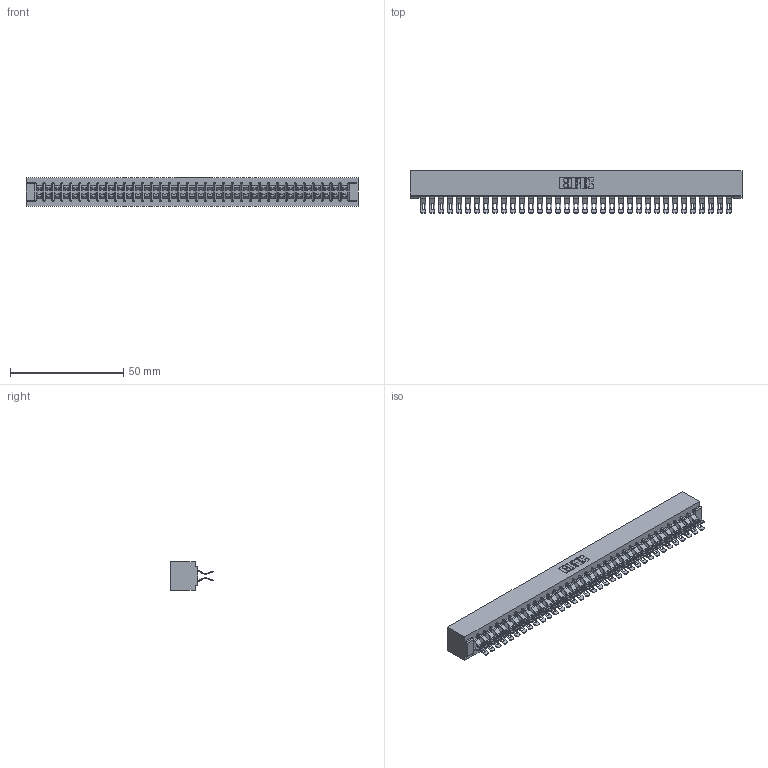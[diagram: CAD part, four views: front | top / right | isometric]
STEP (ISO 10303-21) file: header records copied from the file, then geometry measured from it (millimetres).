
FILE_DESCRIPTION (( 'STEP AP203' ), '1' );
FILE_NAME ('357-070-455-201.STEP', '2020-10-04T21:39:16', ( '' ), ( '' ), 'SwSTEP 2.0', 'SolidWorks 2020', '' );
FILE_SCHEMA (( 'CONFIG_CONTROL_DESIGN' ));
Length unit declared in the file: inch
Products named in the file (3): 307-290-001_555; 307 Part_No Mounting Lugs; 357-070-455-201
Assembly tree (71 placements, depth 2):
  357-070-455-201
    307 Part_No Mounting Lugs
    307-290-001_555  x70
Bounding box: 146.56 x 18.75 x 12.7 mm (x, y, z)
Volume: 16291.2 mm3; surface area: 21264.4 mm2
Topology: 71 solids, 71 shells, 4416 faces, 12969 edges, 8454 vertices
Faces by surface type: plane 2446, cylinder 1898, sphere 72
Entity records: 32247 total; most frequent: CARTESIAN_POINT 5279, ORIENTED_EDGE 5232, DIRECTION 5180, EDGE_CURVE 2616, LINE 1994, VECTOR 1994, VERTEX_POINT 1692, AXIS2_PLACEMENT_3D 1593
